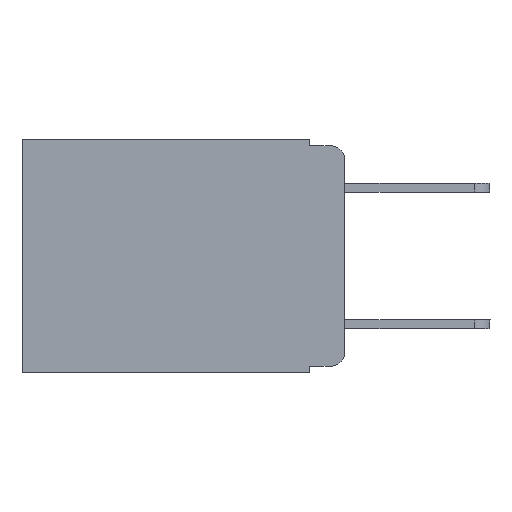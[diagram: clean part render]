
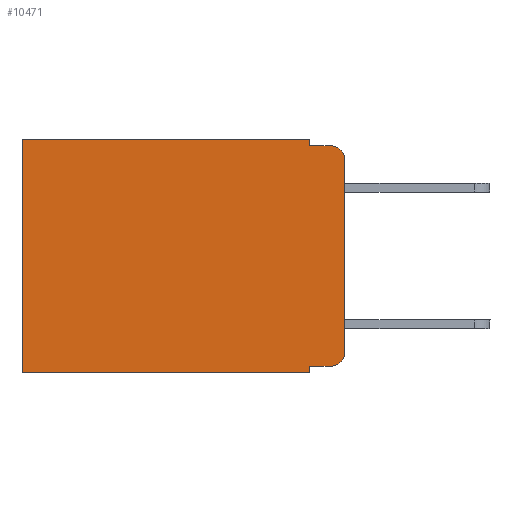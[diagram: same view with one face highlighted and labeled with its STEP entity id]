
A CAD part, left-side view. The second image highlights one B-rep face of the part: STEP entity #10471.
In plain terms, the highlighted planar face has unit normal (-1, 0, 0).
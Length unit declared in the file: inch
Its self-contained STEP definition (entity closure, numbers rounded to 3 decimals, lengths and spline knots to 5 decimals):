
#145 = CARTESIAN_POINT ( 'NONE',  ( 0.298, 0.051, 0. ) ) ;
#153 = CARTESIAN_POINT ( 'NONE',  ( 0.298, 0.051, -0.01 ) ) ;
#240 = EDGE_CURVE ( 'NONE', #8611, #6861, #6200, .T. ) ;
#264 = ORIENTED_EDGE ( 'NONE', *, *, #240, .T. ) ;
#972 = ORIENTED_EDGE ( 'NONE', *, *, #2788, .F. ) ;
#1020 = CARTESIAN_POINT ( 'NONE',  ( 0.298, 0.473, 0. ) ) ;
#1057 = CIRCLE ( 'NONE', #3113, 0.02 ) ;
#1090 = CARTESIAN_POINT ( 'NONE',  ( 0.298, 0., 0. ) ) ;
#1937 = AXIS2_PLACEMENT_3D ( 'NONE', #6667, #15177, #9201 ) ;
#2199 = CARTESIAN_POINT ( 'NONE',  ( 0.298, 0.051, -0.343 ) ) ;
#2291 = DIRECTION ( 'NONE',  ( 0., -1., 0. ) ) ;
#2788 = EDGE_CURVE ( 'NONE', #14857, #14490, #12395, .T. ) ;
#3036 = EDGE_CURVE ( 'NONE', #11021, #6583, #11998, .T. ) ;
#3113 = AXIS2_PLACEMENT_3D ( 'NONE', #13133, #16211, #7353 ) ;
#3154 = LINE ( 'NONE', #145, #14867 ) ;
#3162 = ORIENTED_EDGE ( 'NONE', *, *, #7177, .T. ) ;
#3181 = CARTESIAN_POINT ( 'NONE',  ( 0.298, 0., -0.343 ) ) ;
#3553 = ORIENTED_EDGE ( 'NONE', *, *, #5886, .F. ) ;
#3673 = EDGE_CURVE ( 'NONE', #7133, #12707, #1057, .T. ) ;
#4058 = CARTESIAN_POINT ( 'NONE',  ( 0.298, 0., -0.03 ) ) ;
#4419 = ORIENTED_EDGE ( 'NONE', *, *, #3673, .T. ) ;
#4670 = CARTESIAN_POINT ( 'NONE',  ( 0.298, 0.051, 0. ) ) ;
#4768 = CIRCLE ( 'NONE', #15038, 0.02 ) ;
#4891 = EDGE_CURVE ( 'NONE', #14705, #12707, #14864, .T. ) ;
#4958 = CARTESIAN_POINT ( 'NONE',  ( 0.298, 0.051, -0.333 ) ) ;
#5027 = ORIENTED_EDGE ( 'NONE', *, *, #15175, .T. ) ;
#5208 = EDGE_CURVE ( 'NONE', #6583, #13753, #15258, .T. ) ;
#5240 = CARTESIAN_POINT ( 'NONE',  ( 0.298, 0., 0. ) ) ;
#5393 = DIRECTION ( 'NONE',  ( 0., 0., -1. ) ) ;
#5558 = VECTOR ( 'NONE', #5393, 39.37008 ) ;
#5829 = EDGE_CURVE ( 'NONE', #14705, #14490, #4768, .T. ) ;
#5886 = EDGE_CURVE ( 'NONE', #8611, #14857, #3154, .T. ) ;
#6200 = LINE ( 'NONE', #5240, #15885 ) ;
#6249 = VECTOR ( 'NONE', #9796, 39.37008 ) ;
#6549 = VECTOR ( 'NONE', #9681, 39.37008 ) ;
#6583 = VERTEX_POINT ( 'NONE', #2199 ) ;
#6641 = EDGE_LOOP ( 'NONE', ( #13196, #14753, #972, #3553, #264, #5027, #9530, #9812, #3162, #4419 ) ) ;
#6667 = CARTESIAN_POINT ( 'NONE',  ( 0.298, 0., 0. ) ) ;
#6861 = VERTEX_POINT ( 'NONE', #9056 ) ;
#6887 = VECTOR ( 'NONE', #2291, 39.37008 ) ;
#7133 = VERTEX_POINT ( 'NONE', #14858 ) ;
#7170 = VECTOR ( 'NONE', #8699, 39.37008 ) ;
#7177 = EDGE_CURVE ( 'NONE', #11021, #7133, #12849, .T. ) ;
#7192 = CARTESIAN_POINT ( 'NONE',  ( 0.298, 0., -0.313 ) ) ;
#7199 = CARTESIAN_POINT ( 'NONE',  ( 0.298, 0.02, -0.03 ) ) ;
#7239 = CARTESIAN_POINT ( 'NONE',  ( 0.298, 0.473, -0.343 ) ) ;
#7294 = CARTESIAN_POINT ( 'NONE',  ( 0.298, 0.051, 0. ) ) ;
#7353 = DIRECTION ( 'NONE',  ( 0., 0., -1. ) ) ;
#7806 = CARTESIAN_POINT ( 'NONE',  ( 0.298, 0.051, -0.333 ) ) ;
#8481 = DIRECTION ( 'NONE',  ( 0., 0., -1. ) ) ;
#8611 = VERTEX_POINT ( 'NONE', #4670 ) ;
#8699 = DIRECTION ( 'NONE',  ( 0., 0., -1. ) ) ;
#8780 = FACE_OUTER_BOUND ( 'NONE', #6641, .T. ) ;
#8964 = DIRECTION ( 'NONE',  ( 0., 0., -1. ) ) ;
#9056 = CARTESIAN_POINT ( 'NONE',  ( 0.298, 0.473, 0. ) ) ;
#9201 = DIRECTION ( 'NONE',  ( 0., 0., -1. ) ) ;
#9530 = ORIENTED_EDGE ( 'NONE', *, *, #5208, .F. ) ;
#9681 = DIRECTION ( 'NONE',  ( 0., 1., 0. ) ) ;
#9796 = DIRECTION ( 'NONE',  ( 0., 0., -1. ) ) ;
#9812 = ORIENTED_EDGE ( 'NONE', *, *, #3036, .F. ) ;
#10092 = PLANE ( 'NONE',  #1937 ) ;
#10471 = ADVANCED_FACE ( 'NONE', ( #8780 ), #10092, .F. ) ;
#10788 = VECTOR ( 'NONE', #15397, 39.37008 ) ;
#11021 = VERTEX_POINT ( 'NONE', #7806 ) ;
#11998 = LINE ( 'NONE', #7294, #6249 ) ;
#12395 = LINE ( 'NONE', #153, #10788 ) ;
#12622 = CARTESIAN_POINT ( 'NONE',  ( 0.298, 0.02, -0.01 ) ) ;
#12707 = VERTEX_POINT ( 'NONE', #7192 ) ;
#12849 = LINE ( 'NONE', #4958, #6887 ) ;
#13133 = CARTESIAN_POINT ( 'NONE',  ( 0.298, 0.02, -0.313 ) ) ;
#13196 = ORIENTED_EDGE ( 'NONE', *, *, #4891, .F. ) ;
#13753 = VERTEX_POINT ( 'NONE', #7239 ) ;
#14080 = DIRECTION ( 'NONE',  ( 0., 1., 0. ) ) ;
#14490 = VERTEX_POINT ( 'NONE', #12622 ) ;
#14705 = VERTEX_POINT ( 'NONE', #4058 ) ;
#14753 = ORIENTED_EDGE ( 'NONE', *, *, #5829, .T. ) ;
#14857 = VERTEX_POINT ( 'NONE', #15737 ) ;
#14858 = CARTESIAN_POINT ( 'NONE',  ( 0.298, 0.02, -0.333 ) ) ;
#14864 = LINE ( 'NONE', #1090, #5558 ) ;
#14867 = VECTOR ( 'NONE', #8964, 39.37008 ) ;
#15038 = AXIS2_PLACEMENT_3D ( 'NONE', #7199, #16049, #8481 ) ;
#15175 = EDGE_CURVE ( 'NONE', #6861, #13753, #15499, .T. ) ;
#15177 = DIRECTION ( 'NONE',  ( 1., 0., 0. ) ) ;
#15258 = LINE ( 'NONE', #3181, #6549 ) ;
#15397 = DIRECTION ( 'NONE',  ( 0., -1., 0. ) ) ;
#15499 = LINE ( 'NONE', #1020, #7170 ) ;
#15737 = CARTESIAN_POINT ( 'NONE',  ( 0.298, 0.051, -0.01 ) ) ;
#15885 = VECTOR ( 'NONE', #14080, 39.37008 ) ;
#16049 = DIRECTION ( 'NONE',  ( -1., 0., 0. ) ) ;
#16211 = DIRECTION ( 'NONE',  ( -1., 0., 0. ) ) ;
